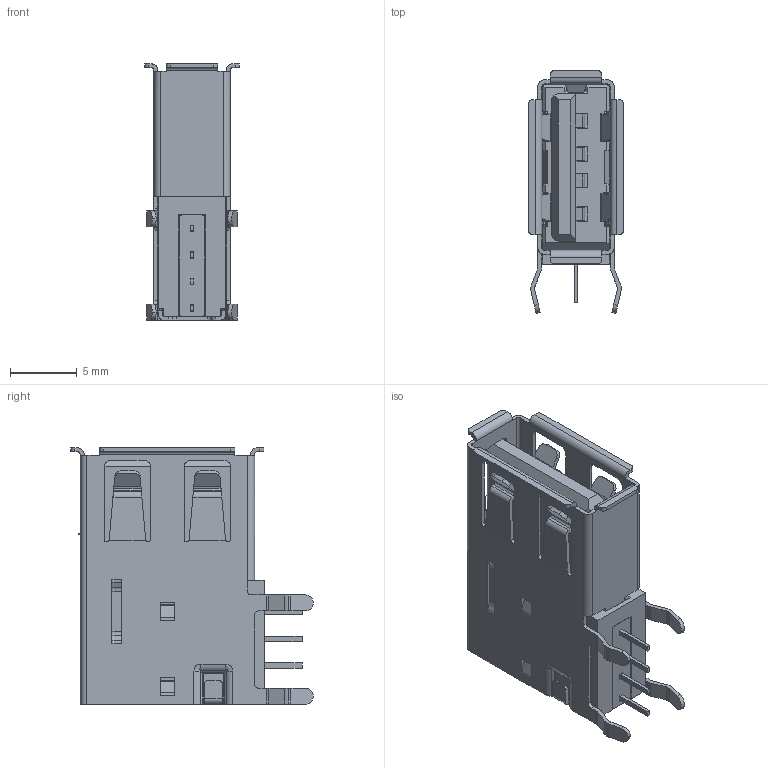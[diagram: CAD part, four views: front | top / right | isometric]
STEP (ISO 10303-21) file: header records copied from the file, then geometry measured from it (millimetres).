
FILE_DESCRIPTION (( 'STEP AP214' ), '1' );
FILE_NAME ('690C104-134-021.STEP', '2021-01-13T22:00:56', ( '' ), ( '' ), 'SwSTEP 2.0', 'SolidWorks 2020', '' );
FILE_SCHEMA (( 'AUTOMOTIVE_DESIGN' ));
Length unit declared in the file: millimetre
Products named in the file (9): Shell 690C104-X34-02X; Contacts_3 690C104-X34-02X; Contacts_4 690C104-X34-02X; Insulator1 690C104-X34-02X_Black; Contacts_1 690C104-X34-02X; 690C104-134-021; Contacts_2 690C104-X34-02X; Contacts 690C104-X34-02X; Insulator2 690C104-X34-02X_White
Assembly tree (8 placements, depth 3):
  690C104-134-021
    Insulator1 690C104-X34-02X_Black
    Contacts 690C104-X34-02X
      Contacts_1 690C104-X34-02X
      Contacts_2 690C104-X34-02X
      Contacts_3 690C104-X34-02X
      Contacts_4 690C104-X34-02X
    Insulator2 690C104-X34-02X_White
    Shell 690C104-X34-02X
Bounding box: 7.12 x 18.2 x 19.25 mm (x, y, z)
Volume: 657.1 mm3; surface area: 2732.9 mm2
Topology: 7 solids, 7 shells, 1141 faces, 3253 edges, 2104 vertices
Faces by surface type: plane 753, cylinder 332, bspline 40, cone 16
Entity records: 39106 total; most frequent: CARTESIAN_POINT 9658, ORIENTED_EDGE 6506, DIRECTION 5497, EDGE_CURVE 3253, LINE 2433, VECTOR 2433, VERTEX_POINT 2104, AXIS2_PLACEMENT_3D 1532
